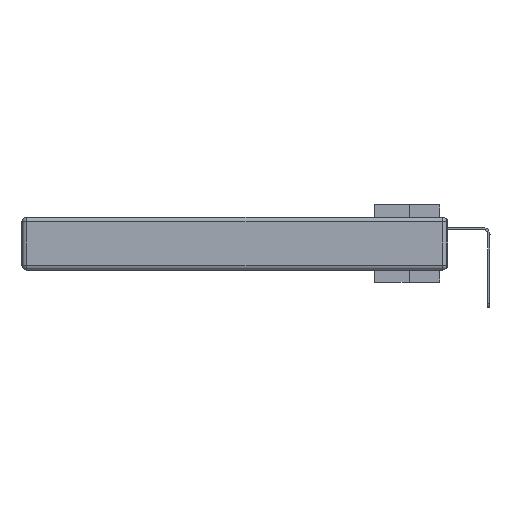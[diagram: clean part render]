
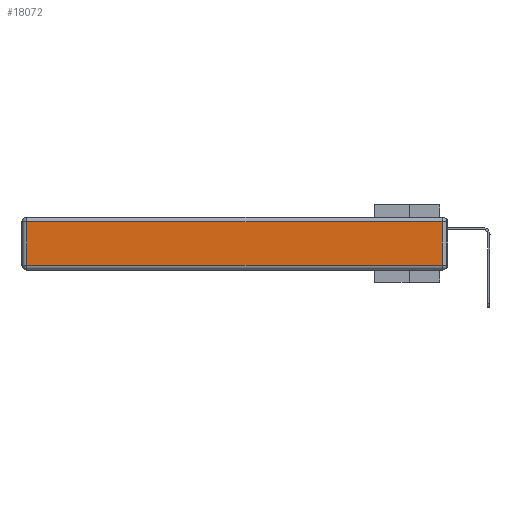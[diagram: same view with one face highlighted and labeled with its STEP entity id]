
A CAD part, left-side view. The second image highlights one B-rep face of the part: STEP entity #18072.
In plain terms, the highlighted planar face has unit normal (-1, 0, 0).
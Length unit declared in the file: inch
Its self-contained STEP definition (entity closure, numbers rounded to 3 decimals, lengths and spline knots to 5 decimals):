
#996 = DIRECTION ( 'NONE',  ( 0., 0., 1. ) ) ;
#1139 = ORIENTED_EDGE ( 'NONE', *, *, #33127, .T. ) ;
#1516 = CARTESIAN_POINT ( 'NONE',  ( 0., 2.72, -0.03 ) ) ;
#2080 = CARTESIAN_POINT ( 'NONE',  ( 0., 2.75, -0.03 ) ) ;
#4234 = VERTEX_POINT ( 'NONE', #18247 ) ;
#5043 = CARTESIAN_POINT ( 'NONE',  ( 0., 2.72, -0.313 ) ) ;
#8285 = LINE ( 'NONE', #2080, #28232 ) ;
#8374 = CARTESIAN_POINT ( 'NONE',  ( 0., 2.72, -0.343 ) ) ;
#9053 = EDGE_LOOP ( 'NONE', ( #1139, #13461, #15819, #22882 ) ) ;
#9680 = AXIS2_PLACEMENT_3D ( 'NONE', #15127, #17511, #34166 ) ;
#11117 = DIRECTION ( 'NONE',  ( 0., 0., -1. ) ) ;
#11541 = LINE ( 'NONE', #24611, #17057 ) ;
#13065 = VERTEX_POINT ( 'NONE', #24898 ) ;
#13461 = ORIENTED_EDGE ( 'NONE', *, *, #29941, .T. ) ;
#15127 = CARTESIAN_POINT ( 'NONE',  ( 0., 0., -0.343 ) ) ;
#15819 = ORIENTED_EDGE ( 'NONE', *, *, #25650, .T. ) ;
#16235 = VERTEX_POINT ( 'NONE', #1516 ) ;
#17057 = VECTOR ( 'NONE', #27104, 39.37008 ) ;
#17457 = CARTESIAN_POINT ( 'NONE',  ( 0., 0.03, -0.343 ) ) ;
#17511 = DIRECTION ( 'NONE',  ( -1., 0., 0. ) ) ;
#18072 = ADVANCED_FACE ( 'NONE', ( #21303 ), #28666, .T. ) ;
#18247 = CARTESIAN_POINT ( 'NONE',  ( 0., 0.03, -0.313 ) ) ;
#21303 = FACE_OUTER_BOUND ( 'NONE', #9053, .T. ) ;
#22882 = ORIENTED_EDGE ( 'NONE', *, *, #24107, .T. ) ;
#24107 = EDGE_CURVE ( 'NONE', #16235, #27113, #25771, .T. ) ;
#24611 = CARTESIAN_POINT ( 'NONE',  ( 0., 0., -0.313 ) ) ;
#24898 = CARTESIAN_POINT ( 'NONE',  ( 0., 0.03, -0.03 ) ) ;
#25650 = EDGE_CURVE ( 'NONE', #13065, #16235, #8285, .T. ) ;
#25771 = LINE ( 'NONE', #8374, #29612 ) ;
#26433 = LINE ( 'NONE', #17457, #32834 ) ;
#27104 = DIRECTION ( 'NONE',  ( 0., -1., 0. ) ) ;
#27113 = VERTEX_POINT ( 'NONE', #5043 ) ;
#28232 = VECTOR ( 'NONE', #31631, 39.37008 ) ;
#28666 = PLANE ( 'NONE',  #9680 ) ;
#29612 = VECTOR ( 'NONE', #11117, 39.37008 ) ;
#29941 = EDGE_CURVE ( 'NONE', #4234, #13065, #26433, .T. ) ;
#31631 = DIRECTION ( 'NONE',  ( 0., 1., 0. ) ) ;
#32834 = VECTOR ( 'NONE', #996, 39.37008 ) ;
#33127 = EDGE_CURVE ( 'NONE', #27113, #4234, #11541, .T. ) ;
#34166 = DIRECTION ( 'NONE',  ( 0., 0., 1. ) ) ;
